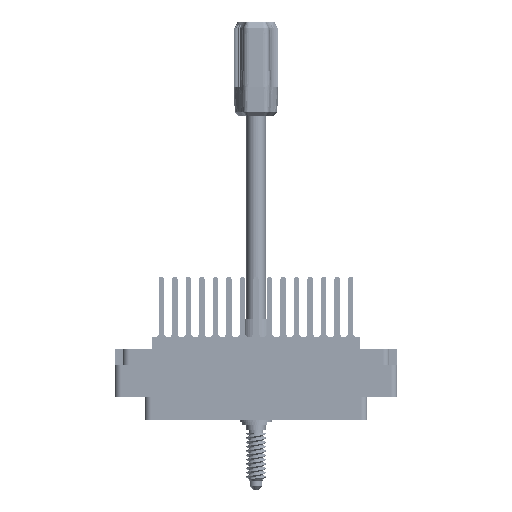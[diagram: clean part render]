
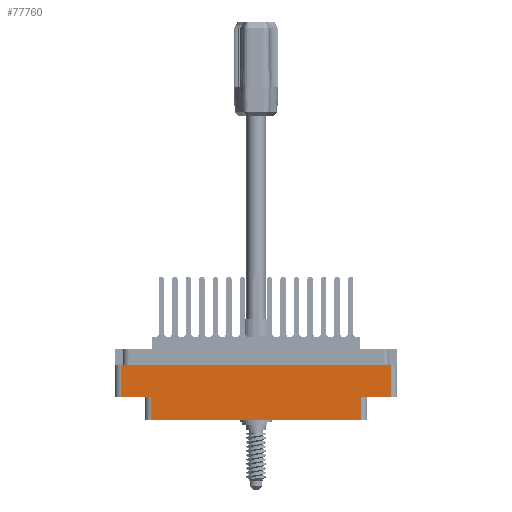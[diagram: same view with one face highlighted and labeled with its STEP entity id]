
A CAD part, front view. The second image highlights one B-rep face of the part: STEP entity #77760.
In plain terms, the highlighted planar face has unit normal (0, -1, 0).
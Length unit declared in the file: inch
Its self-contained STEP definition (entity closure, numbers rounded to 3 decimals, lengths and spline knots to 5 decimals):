
#470 = VECTOR ( 'NONE', #7098, 39.37008 ) ;
#502 = PLANE ( 'NONE',  #83464 ) ;
#2664 = ORIENTED_EDGE ( 'NONE', *, *, #37136, .T. ) ;
#3139 = VECTOR ( 'NONE', #41552, 39.37008 ) ;
#4204 = DIRECTION ( 'NONE',  ( 1., 0., 0. ) ) ;
#5018 = CARTESIAN_POINT ( 'NONE',  ( 1.297, -0.617, -0.798 ) ) ;
#5783 = VERTEX_POINT ( 'NONE', #12327 ) ;
#7098 = DIRECTION ( 'NONE',  ( 0., 0., -1. ) ) ;
#7137 = EDGE_CURVE ( 'NONE', #24444, #59189, #33379, .T. ) ;
#10638 = CARTESIAN_POINT ( 'NONE',  ( 1.006, -0.617, -0.578 ) ) ;
#11852 = CARTESIAN_POINT ( 'NONE',  ( -1.297, -0.617, -0.578 ) ) ;
#12090 = EDGE_LOOP ( 'NONE', ( #12761, #25203, #71899, #23775, #72480, #2664, #51146, #57895 ) ) ;
#12264 = EDGE_CURVE ( 'NONE', #5783, #40729, #41830, .T. ) ;
#12327 = CARTESIAN_POINT ( 'NONE',  ( -1.006, -0.617, -0.798 ) ) ;
#12761 = ORIENTED_EDGE ( 'NONE', *, *, #70229, .T. ) ;
#13105 = DIRECTION ( 'NONE',  ( 0., 0., -1. ) ) ;
#15492 = VERTEX_POINT ( 'NONE', #19912 ) ;
#16587 = DIRECTION ( 'NONE',  ( 0., 0., 1. ) ) ;
#19912 = CARTESIAN_POINT ( 'NONE',  ( 1.297, -0.617, -0.274 ) ) ;
#20126 = VECTOR ( 'NONE', #4204, 39.37008 ) ;
#20662 = CARTESIAN_POINT ( 'NONE',  ( 1.297, -0.617, -0.578 ) ) ;
#20836 = CARTESIAN_POINT ( 'NONE',  ( -1.297, -0.617, -0.274 ) ) ;
#23364 = VERTEX_POINT ( 'NONE', #20662 ) ;
#23775 = ORIENTED_EDGE ( 'NONE', *, *, #82842, .T. ) ;
#24227 = LINE ( 'NONE', #43167, #20126 ) ;
#24444 = VERTEX_POINT ( 'NONE', #20836 ) ;
#25203 = ORIENTED_EDGE ( 'NONE', *, *, #72449, .T. ) ;
#27112 = VECTOR ( 'NONE', #83569, 39.37008 ) ;
#27744 = CARTESIAN_POINT ( 'NONE',  ( 1.006, -0.617, -0.578 ) ) ;
#30347 = LINE ( 'NONE', #10638, #59954 ) ;
#32159 = DIRECTION ( 'NONE',  ( -1., 0., 0. ) ) ;
#33345 = VERTEX_POINT ( 'NONE', #27744 ) ;
#33379 = LINE ( 'NONE', #65540, #52763 ) ;
#37136 = EDGE_CURVE ( 'NONE', #23364, #15492, #61799, .T. ) ;
#40729 = VERTEX_POINT ( 'NONE', #54122 ) ;
#41552 = DIRECTION ( 'NONE',  ( 1., 0., 0. ) ) ;
#41642 = VECTOR ( 'NONE', #45694, 39.37008 ) ;
#41830 = LINE ( 'NONE', #61528, #3139 ) ;
#43167 = CARTESIAN_POINT ( 'NONE',  ( 0., -0.617, -0.274 ) ) ;
#45694 = DIRECTION ( 'NONE',  ( 1., 0., 0. ) ) ;
#46083 = CARTESIAN_POINT ( 'NONE',  ( -1.006, -0.617, -0.798 ) ) ;
#46084 = DIRECTION ( 'NONE',  ( 0., 0., -1. ) ) ;
#46532 = CARTESIAN_POINT ( 'NONE',  ( -1.006, -0.617, -0.578 ) ) ;
#46642 = DIRECTION ( 'NONE',  ( 0., -1., 0. ) ) ;
#49407 = LINE ( 'NONE', #46083, #470 ) ;
#51146 = ORIENTED_EDGE ( 'NONE', *, *, #77891, .F. ) ;
#51506 = CARTESIAN_POINT ( 'NONE',  ( 0., -0.617, -0.578 ) ) ;
#52763 = VECTOR ( 'NONE', #13105, 39.37008 ) ;
#54122 = CARTESIAN_POINT ( 'NONE',  ( 1.006, -0.617, -0.798 ) ) ;
#55908 = FACE_OUTER_BOUND ( 'NONE', #12090, .T. ) ;
#57895 = ORIENTED_EDGE ( 'NONE', *, *, #7137, .T. ) ;
#59189 = VERTEX_POINT ( 'NONE', #11852 ) ;
#59954 = VECTOR ( 'NONE', #16587, 39.37008 ) ;
#59963 = VECTOR ( 'NONE', #32159, 39.37008 ) ;
#61528 = CARTESIAN_POINT ( 'NONE',  ( -1.359, -0.617, -0.798 ) ) ;
#61799 = LINE ( 'NONE', #5018, #27112 ) ;
#65540 = CARTESIAN_POINT ( 'NONE',  ( -1.297, -0.617, -0.798 ) ) ;
#66311 = CARTESIAN_POINT ( 'NONE',  ( -1.359, -0.617, -0.798 ) ) ;
#70229 = EDGE_CURVE ( 'NONE', #59189, #74920, #75296, .T. ) ;
#71899 = ORIENTED_EDGE ( 'NONE', *, *, #12264, .T. ) ;
#72449 = EDGE_CURVE ( 'NONE', #74920, #5783, #49407, .T. ) ;
#72465 = CARTESIAN_POINT ( 'NONE',  ( 0., -0.617, -0.578 ) ) ;
#72480 = ORIENTED_EDGE ( 'NONE', *, *, #77679, .F. ) ;
#74920 = VERTEX_POINT ( 'NONE', #46532 ) ;
#75296 = LINE ( 'NONE', #72465, #41642 ) ;
#77245 = LINE ( 'NONE', #51506, #59963 ) ;
#77679 = EDGE_CURVE ( 'NONE', #23364, #33345, #77245, .T. ) ;
#77760 = ADVANCED_FACE ( 'NONE', ( #55908 ), #502, .T. ) ;
#77891 = EDGE_CURVE ( 'NONE', #24444, #15492, #24227, .T. ) ;
#82842 = EDGE_CURVE ( 'NONE', #40729, #33345, #30347, .T. ) ;
#83464 = AXIS2_PLACEMENT_3D ( 'NONE', #66311, #46642, #46084 ) ;
#83569 = DIRECTION ( 'NONE',  ( 0., 0., 1. ) ) ;
